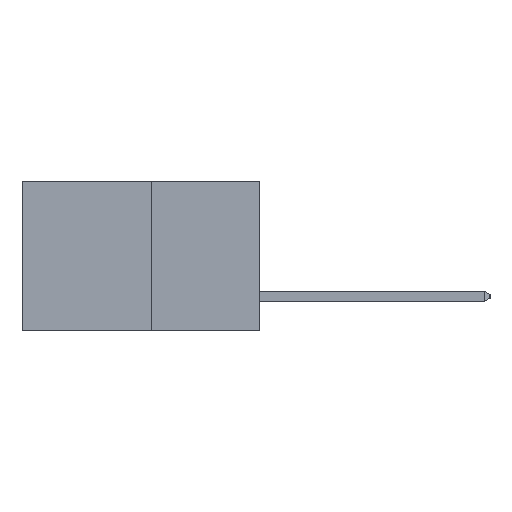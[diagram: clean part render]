
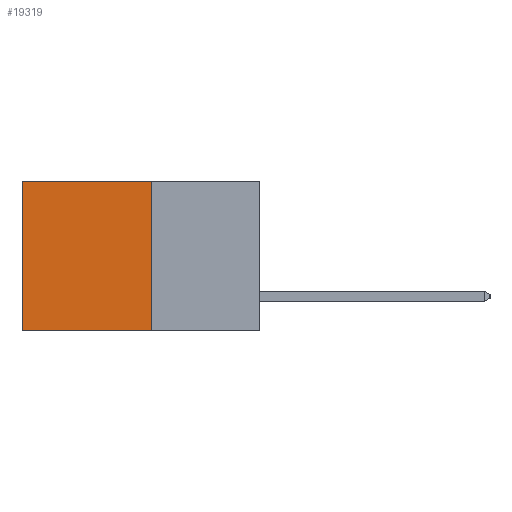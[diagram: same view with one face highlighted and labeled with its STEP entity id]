
A CAD part, left-side view. The second image highlights one B-rep face of the part: STEP entity #19319.
In plain terms, the highlighted planar face has unit normal (-1, 0, 0).
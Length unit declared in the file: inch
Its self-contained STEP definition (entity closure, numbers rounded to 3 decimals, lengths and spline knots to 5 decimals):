
#1094 = CARTESIAN_POINT ( 'NONE',  ( 0.277, 0.27, -0.37 ) ) ;
#1517 = VECTOR ( 'NONE', #13572, 39.37008 ) ;
#1642 = ORIENTED_EDGE ( 'NONE', *, *, #12724, .T. ) ;
#2763 = EDGE_CURVE ( 'NONE', #14141, #20470, #18764, .T. ) ;
#4479 = ORIENTED_EDGE ( 'NONE', *, *, #2763, .T. ) ;
#5903 = ORIENTED_EDGE ( 'NONE', *, *, #21678, .F. ) ;
#6715 = CARTESIAN_POINT ( 'NONE',  ( 0.277, 0.59, -0.37 ) ) ;
#7509 = DIRECTION ( 'NONE',  ( 1., 0., 0. ) ) ;
#7881 = DIRECTION ( 'NONE',  ( 0., 1., 0. ) ) ;
#8101 = EDGE_LOOP ( 'NONE', ( #4479, #23680, #5903, #1642 ) ) ;
#8707 = VECTOR ( 'NONE', #10523, 39.37008 ) ;
#10264 = CARTESIAN_POINT ( 'NONE',  ( 0.277, 0.27, -0.37 ) ) ;
#10441 = CARTESIAN_POINT ( 'NONE',  ( 0.277, 0.27, -0.37 ) ) ;
#10523 = DIRECTION ( 'NONE',  ( 0., 1., 0. ) ) ;
#10606 = CARTESIAN_POINT ( 'NONE',  ( 0.277, 0.59, -0.37 ) ) ;
#12518 = VECTOR ( 'NONE', #7881, 39.37008 ) ;
#12724 = EDGE_CURVE ( 'NONE', #13935, #14141, #13182, .T. ) ;
#13182 = LINE ( 'NONE', #22341, #12518 ) ;
#13509 = CARTESIAN_POINT ( 'NONE',  ( 0.277, 0.27, 0. ) ) ;
#13572 = DIRECTION ( 'NONE',  ( 0., 0., -1. ) ) ;
#13935 = VERTEX_POINT ( 'NONE', #13509 ) ;
#14141 = VERTEX_POINT ( 'NONE', #22286 ) ;
#15818 = CARTESIAN_POINT ( 'NONE',  ( 0.277, 0.27, -0.37 ) ) ;
#16549 = DIRECTION ( 'NONE',  ( 0., 0., -1. ) ) ;
#18445 = LINE ( 'NONE', #10441, #8707 ) ;
#18764 = LINE ( 'NONE', #10606, #1517 ) ;
#19319 = ADVANCED_FACE ( 'NONE', ( #26198 ), #19932, .F. ) ;
#19932 = PLANE ( 'NONE',  #22660 ) ;
#20470 = VERTEX_POINT ( 'NONE', #6715 ) ;
#21678 = EDGE_CURVE ( 'NONE', #13935, #24649, #25762, .T. ) ;
#21991 = DIRECTION ( 'NONE',  ( 0., 0., -1. ) ) ;
#22286 = CARTESIAN_POINT ( 'NONE',  ( 0.277, 0.59, 0. ) ) ;
#22341 = CARTESIAN_POINT ( 'NONE',  ( 0.277, 0.27, 0. ) ) ;
#22660 = AXIS2_PLACEMENT_3D ( 'NONE', #15818, #7509, #21991 ) ;
#23597 = EDGE_CURVE ( 'NONE', #24649, #20470, #18445, .T. ) ;
#23680 = ORIENTED_EDGE ( 'NONE', *, *, #23597, .F. ) ;
#24649 = VERTEX_POINT ( 'NONE', #1094 ) ;
#25152 = VECTOR ( 'NONE', #16549, 39.37008 ) ;
#25762 = LINE ( 'NONE', #10264, #25152 ) ;
#26198 = FACE_OUTER_BOUND ( 'NONE', #8101, .T. ) ;
